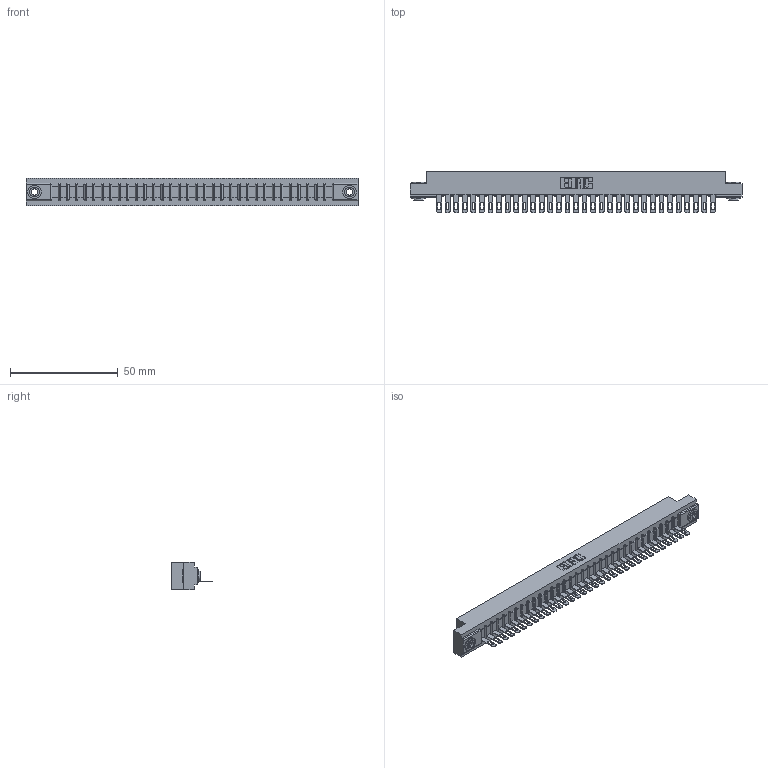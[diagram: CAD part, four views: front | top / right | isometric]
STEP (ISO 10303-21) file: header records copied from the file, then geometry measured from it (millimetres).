
FILE_DESCRIPTION (( 'STEP AP203' ), '1' );
FILE_NAME ('307-033-405-103.STEP', '2020-09-28T17:20:01', ( '' ), ( '' ), 'SwSTEP 2.0', 'SolidWorks 2020', '' );
FILE_SCHEMA (( 'CONFIG_CONTROL_DESIGN' ));
Length unit declared in the file: inch
Products named in the file (4): 307-290-001_505; 307-033-405-103; 307 Part_.156 Dia Mounting Holes; 345-250-002_345-250-002-102
Assembly tree (36 placements, depth 2):
  307-033-405-103
    307 Part_.156 Dia Mounting Holes
    307-290-001_505  x33
    345-250-002_345-250-002-102  x2
Bounding box: 153.77 x 19.18 x 12.7 mm (x, y, z)
Volume: 15958.1 mm3; surface area: 17324.6 mm2
Topology: 36 solids, 36 shells, 2052 faces, 5781 edges, 3714 vertices
Faces by surface type: plane 1282, cylinder 694, sphere 68, cone 8
Entity records: 30439 total; most frequent: CARTESIAN_POINT 5101, ORIENTED_EDGE 5078, DIRECTION 4983, EDGE_CURVE 2539, VECTOR 1935, LINE 1935, VERTEX_POINT 1642, AXIS2_PLACEMENT_3D 1524
